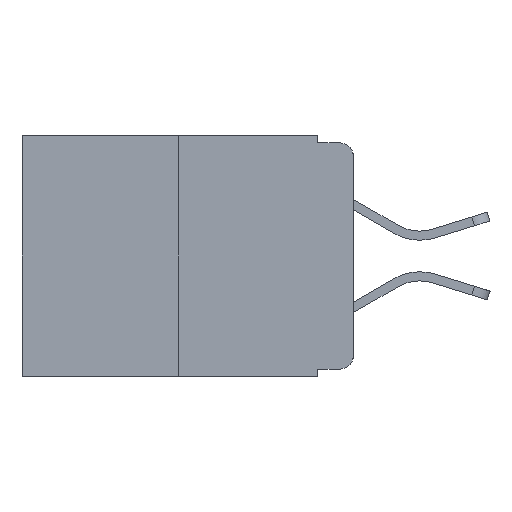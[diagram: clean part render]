
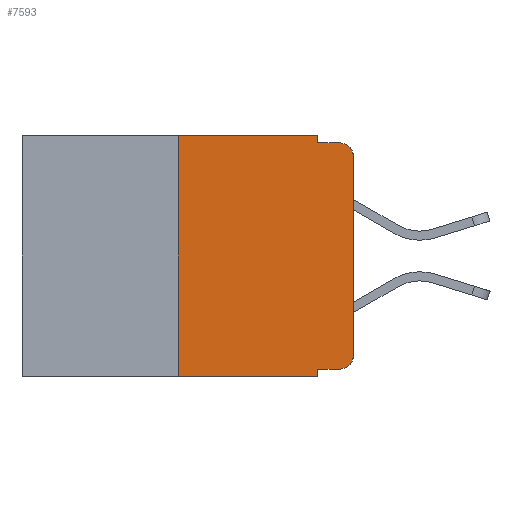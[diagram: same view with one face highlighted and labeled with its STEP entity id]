
A CAD part, left-side view. The second image highlights one B-rep face of the part: STEP entity #7593.
In plain terms, the highlighted planar face has unit normal (-1, 0, 0).
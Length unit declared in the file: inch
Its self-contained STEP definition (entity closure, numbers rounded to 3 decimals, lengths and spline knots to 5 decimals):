
#421 = VERTEX_POINT ( 'NONE', #6680 ) ;
#834 = VERTEX_POINT ( 'NONE', #10276 ) ;
#1004 = EDGE_CURVE ( 'NONE', #1357, #10119, #2474, .T. ) ;
#1063 = CARTESIAN_POINT ( 'NONE',  ( 0., 0., -0.313 ) ) ;
#1179 = DIRECTION ( 'NONE',  ( 0., 0., -1. ) ) ;
#1357 = VERTEX_POINT ( 'NONE', #11603 ) ;
#1683 = VERTEX_POINT ( 'NONE', #2451 ) ;
#1687 = VECTOR ( 'NONE', #12033, 39.37008 ) ;
#1858 = CARTESIAN_POINT ( 'NONE',  ( 0., 0., -0.03 ) ) ;
#1906 = ORIENTED_EDGE ( 'NONE', *, *, #7242, .F. ) ;
#2016 = ORIENTED_EDGE ( 'NONE', *, *, #12669, .T. ) ;
#2118 = ORIENTED_EDGE ( 'NONE', *, *, #4551, .T. ) ;
#2222 = CARTESIAN_POINT ( 'NONE',  ( 0., 0.25, 0. ) ) ;
#2388 = DIRECTION ( 'NONE',  ( 0., 0., 1. ) ) ;
#2451 = CARTESIAN_POINT ( 'NONE',  ( 0., 0.25, -0.343 ) ) ;
#2474 = CIRCLE ( 'NONE', #11857, 0.02 ) ;
#2501 = VECTOR ( 'NONE', #13991, 39.37008 ) ;
#2774 = EDGE_CURVE ( 'NONE', #834, #421, #3625, .T. ) ;
#3248 = LINE ( 'NONE', #4345, #9934 ) ;
#3377 = CARTESIAN_POINT ( 'NONE',  ( 0., 0.051, 0. ) ) ;
#3522 = DIRECTION ( 'NONE',  ( 0., -1., 0. ) ) ;
#3625 = LINE ( 'NONE', #3377, #11370 ) ;
#3666 = EDGE_CURVE ( 'NONE', #9542, #9537, #10268, .T. ) ;
#3708 = DIRECTION ( 'NONE',  ( 1., 0., 0. ) ) ;
#3784 = ORIENTED_EDGE ( 'NONE', *, *, #9306, .F. ) ;
#4345 = CARTESIAN_POINT ( 'NONE',  ( 0., 0.473, 0. ) ) ;
#4502 = CARTESIAN_POINT ( 'NONE',  ( 0., 0.051, -0.01 ) ) ;
#4548 = VERTEX_POINT ( 'NONE', #2222 ) ;
#4551 = EDGE_CURVE ( 'NONE', #1683, #421, #11686, .T. ) ;
#4858 = EDGE_CURVE ( 'NONE', #10119, #9542, #6891, .T. ) ;
#4946 = DIRECTION ( 'NONE',  ( -1., 0., 0. ) ) ;
#4990 = LINE ( 'NONE', #10433, #14702 ) ;
#5013 = PLANE ( 'NONE',  #11410 ) ;
#5407 = VECTOR ( 'NONE', #11520, 39.37008 ) ;
#5573 = VERTEX_POINT ( 'NONE', #14177 ) ;
#5587 = ORIENTED_EDGE ( 'NONE', *, *, #3666, .T. ) ;
#5670 = DIRECTION ( 'NONE',  ( 0., 0., -1. ) ) ;
#5739 = CARTESIAN_POINT ( 'NONE',  ( 0., 0.25, 0. ) ) ;
#5910 = DIRECTION ( 'NONE',  ( 0., 0., -1. ) ) ;
#6250 = VERTEX_POINT ( 'NONE', #10778 ) ;
#6680 = CARTESIAN_POINT ( 'NONE',  ( 0., 0.051, -0.343 ) ) ;
#6728 = CARTESIAN_POINT ( 'NONE',  ( 0., 0.051, 0. ) ) ;
#6891 = LINE ( 'NONE', #12121, #1687 ) ;
#6998 = DIRECTION ( 'NONE',  ( 0., 0., -1. ) ) ;
#7242 = EDGE_CURVE ( 'NONE', #6250, #5573, #10474, .T. ) ;
#7543 = ORIENTED_EDGE ( 'NONE', *, *, #11941, .F. ) ;
#7593 = ADVANCED_FACE ( 'NONE', ( #14039 ), #5013, .F. ) ;
#7666 = DIRECTION ( 'NONE',  ( 0., -1., 0. ) ) ;
#7890 = AXIS2_PLACEMENT_3D ( 'NONE', #14048, #4946, #13012 ) ;
#8107 = DIRECTION ( 'NONE',  ( -1., 0., 0. ) ) ;
#8355 = ORIENTED_EDGE ( 'NONE', *, *, #9710, .F. ) ;
#8387 = EDGE_LOOP ( 'NONE', ( #12406, #5587, #3784, #1906, #8355, #7543, #2118, #14444, #2016, #14813 ) ) ;
#9306 = EDGE_CURVE ( 'NONE', #5573, #9537, #14415, .T. ) ;
#9537 = VERTEX_POINT ( 'NONE', #13424 ) ;
#9542 = VERTEX_POINT ( 'NONE', #1858 ) ;
#9710 = EDGE_CURVE ( 'NONE', #4548, #6250, #3248, .T. ) ;
#9893 = LINE ( 'NONE', #5739, #11698 ) ;
#9934 = VECTOR ( 'NONE', #7666, 39.37008 ) ;
#10045 = CARTESIAN_POINT ( 'NONE',  ( 0., 0.02, -0.313 ) ) ;
#10119 = VERTEX_POINT ( 'NONE', #1063 ) ;
#10268 = CIRCLE ( 'NONE', #7890, 0.02 ) ;
#10276 = CARTESIAN_POINT ( 'NONE',  ( 0., 0.051, -0.333 ) ) ;
#10433 = CARTESIAN_POINT ( 'NONE',  ( 0., 0.051, -0.333 ) ) ;
#10474 = LINE ( 'NONE', #6728, #11349 ) ;
#10778 = CARTESIAN_POINT ( 'NONE',  ( 0., 0.051, 0. ) ) ;
#11349 = VECTOR ( 'NONE', #5670, 39.37008 ) ;
#11370 = VECTOR ( 'NONE', #6998, 39.37008 ) ;
#11410 = AXIS2_PLACEMENT_3D ( 'NONE', #13033, #3708, #5910 ) ;
#11520 = DIRECTION ( 'NONE',  ( 0., -1., 0. ) ) ;
#11603 = CARTESIAN_POINT ( 'NONE',  ( 0., 0.02, -0.333 ) ) ;
#11686 = LINE ( 'NONE', #11855, #2501 ) ;
#11698 = VECTOR ( 'NONE', #2388, 39.37008 ) ;
#11855 = CARTESIAN_POINT ( 'NONE',  ( 0., 0.473, -0.343 ) ) ;
#11857 = AXIS2_PLACEMENT_3D ( 'NONE', #10045, #8107, #1179 ) ;
#11941 = EDGE_CURVE ( 'NONE', #1683, #4548, #9893, .T. ) ;
#12033 = DIRECTION ( 'NONE',  ( 0., 0., 1. ) ) ;
#12121 = CARTESIAN_POINT ( 'NONE',  ( 0., 0., 0. ) ) ;
#12406 = ORIENTED_EDGE ( 'NONE', *, *, #4858, .T. ) ;
#12669 = EDGE_CURVE ( 'NONE', #834, #1357, #4990, .T. ) ;
#13012 = DIRECTION ( 'NONE',  ( 0., 0., -1. ) ) ;
#13033 = CARTESIAN_POINT ( 'NONE',  ( 0., 0.473, 0. ) ) ;
#13424 = CARTESIAN_POINT ( 'NONE',  ( 0., 0.02, -0.01 ) ) ;
#13991 = DIRECTION ( 'NONE',  ( 0., -1., 0. ) ) ;
#14039 = FACE_OUTER_BOUND ( 'NONE', #8387, .T. ) ;
#14048 = CARTESIAN_POINT ( 'NONE',  ( 0., 0.02, -0.03 ) ) ;
#14177 = CARTESIAN_POINT ( 'NONE',  ( 0., 0.051, -0.01 ) ) ;
#14415 = LINE ( 'NONE', #4502, #5407 ) ;
#14444 = ORIENTED_EDGE ( 'NONE', *, *, #2774, .F. ) ;
#14702 = VECTOR ( 'NONE', #3522, 39.37008 ) ;
#14813 = ORIENTED_EDGE ( 'NONE', *, *, #1004, .T. ) ;
